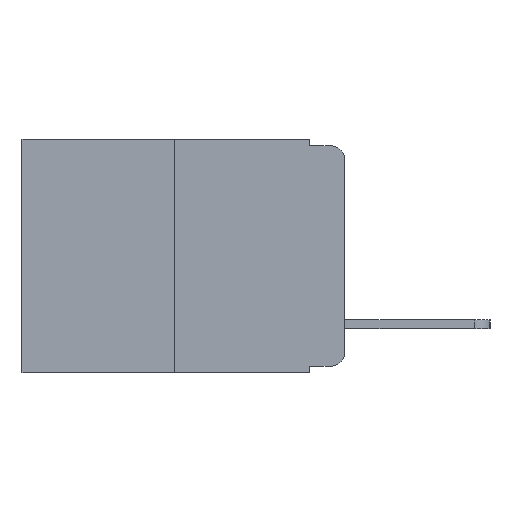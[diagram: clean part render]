
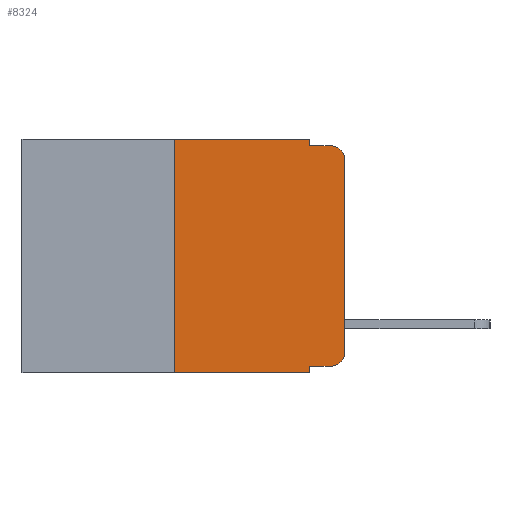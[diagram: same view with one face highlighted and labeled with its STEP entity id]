
A CAD part, left-side view. The second image highlights one B-rep face of the part: STEP entity #8324.
In plain terms, the highlighted planar face has unit normal (-1, 0, 0).
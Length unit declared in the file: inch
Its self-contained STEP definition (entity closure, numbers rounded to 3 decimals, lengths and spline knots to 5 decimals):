
#100 = CARTESIAN_POINT ( 'NONE',  ( 0., 0.051, -0.333 ) ) ;
#491 = VERTEX_POINT ( 'NONE', #8884 ) ;
#670 = VERTEX_POINT ( 'NONE', #9890 ) ;
#972 = VECTOR ( 'NONE', #1448, 39.37008 ) ;
#1049 = EDGE_CURVE ( 'NONE', #491, #8354, #5677, .T. ) ;
#1166 = LINE ( 'NONE', #12088, #6371 ) ;
#1448 = DIRECTION ( 'NONE',  ( 0., 0., 1. ) ) ;
#1479 = VECTOR ( 'NONE', #1860, 39.37008 ) ;
#1709 = PLANE ( 'NONE',  #5831 ) ;
#1791 = VERTEX_POINT ( 'NONE', #10513 ) ;
#1794 = VECTOR ( 'NONE', #8146, 39.37008 ) ;
#1860 = DIRECTION ( 'NONE',  ( 0., -1., 0. ) ) ;
#1942 = AXIS2_PLACEMENT_3D ( 'NONE', #11087, #5425, #11961 ) ;
#1957 = VECTOR ( 'NONE', #8129, 39.37008 ) ;
#1974 = EDGE_CURVE ( 'NONE', #1791, #10375, #2445, .T. ) ;
#2292 = LINE ( 'NONE', #7148, #12209 ) ;
#2402 = LINE ( 'NONE', #7949, #9971 ) ;
#2424 = ORIENTED_EDGE ( 'NONE', *, *, #10102, .T. ) ;
#2445 = CIRCLE ( 'NONE', #5504, 0.02 ) ;
#2684 = EDGE_CURVE ( 'NONE', #4507, #1791, #2402, .T. ) ;
#2780 = DIRECTION ( 'NONE',  ( 0., 0., -1. ) ) ;
#2944 = ORIENTED_EDGE ( 'NONE', *, *, #4035, .F. ) ;
#2957 = VECTOR ( 'NONE', #10579, 39.37008 ) ;
#3113 = DIRECTION ( 'NONE',  ( 0., 0., -1. ) ) ;
#3202 = ORIENTED_EDGE ( 'NONE', *, *, #3351, .F. ) ;
#3351 = EDGE_CURVE ( 'NONE', #4507, #4591, #1166, .T. ) ;
#3646 = ORIENTED_EDGE ( 'NONE', *, *, #1049, .F. ) ;
#3721 = ORIENTED_EDGE ( 'NONE', *, *, #11720, .T. ) ;
#3833 = CARTESIAN_POINT ( 'NONE',  ( 0., 0.051, 0. ) ) ;
#4035 = EDGE_CURVE ( 'NONE', #6986, #491, #11165, .T. ) ;
#4389 = CARTESIAN_POINT ( 'NONE',  ( 0., 0.02, -0.313 ) ) ;
#4422 = CARTESIAN_POINT ( 'NONE',  ( 0., 0., -0.313 ) ) ;
#4507 = VERTEX_POINT ( 'NONE', #100 ) ;
#4591 = VERTEX_POINT ( 'NONE', #7546 ) ;
#5425 = DIRECTION ( 'NONE',  ( -1., 0., 0. ) ) ;
#5504 = AXIS2_PLACEMENT_3D ( 'NONE', #4389, #8541, #8479 ) ;
#5677 = LINE ( 'NONE', #8475, #2957 ) ;
#5831 = AXIS2_PLACEMENT_3D ( 'NONE', #11436, #8782, #2780 ) ;
#6112 = EDGE_CURVE ( 'NONE', #8354, #11029, #2292, .T. ) ;
#6114 = ORIENTED_EDGE ( 'NONE', *, *, #2684, .T. ) ;
#6132 = ORIENTED_EDGE ( 'NONE', *, *, #8092, .T. ) ;
#6163 = CARTESIAN_POINT ( 'NONE',  ( 0., 0.051, -0.01 ) ) ;
#6369 = ORIENTED_EDGE ( 'NONE', *, *, #1974, .T. ) ;
#6371 = VECTOR ( 'NONE', #10505, 39.37008 ) ;
#6565 = DIRECTION ( 'NONE',  ( 0., -1., 0. ) ) ;
#6590 = CARTESIAN_POINT ( 'NONE',  ( 0., 0.25, 0. ) ) ;
#6633 = LINE ( 'NONE', #12437, #1479 ) ;
#6772 = EDGE_CURVE ( 'NONE', #11029, #670, #9754, .T. ) ;
#6856 = EDGE_LOOP ( 'NONE', ( #3721, #6132, #10004, #7521, #3646, #2944, #2424, #3202, #6114, #6369 ) ) ;
#6986 = VERTEX_POINT ( 'NONE', #11988 ) ;
#7148 = CARTESIAN_POINT ( 'NONE',  ( 0., 0.051, 0. ) ) ;
#7205 = CIRCLE ( 'NONE', #1942, 0.02 ) ;
#7376 = LINE ( 'NONE', #9073, #1957 ) ;
#7521 = ORIENTED_EDGE ( 'NONE', *, *, #6112, .F. ) ;
#7546 = CARTESIAN_POINT ( 'NONE',  ( 0., 0.051, -0.343 ) ) ;
#7949 = CARTESIAN_POINT ( 'NONE',  ( 0., 0.051, -0.333 ) ) ;
#8092 = EDGE_CURVE ( 'NONE', #12553, #670, #7205, .T. ) ;
#8129 = DIRECTION ( 'NONE',  ( 0., 0., 1. ) ) ;
#8146 = DIRECTION ( 'NONE',  ( 0., -1., 0. ) ) ;
#8324 = ADVANCED_FACE ( 'NONE', ( #11644 ), #1709, .F. ) ;
#8354 = VERTEX_POINT ( 'NONE', #3833 ) ;
#8475 = CARTESIAN_POINT ( 'NONE',  ( 0., 0.473, 0. ) ) ;
#8479 = DIRECTION ( 'NONE',  ( 0., 0., -1. ) ) ;
#8541 = DIRECTION ( 'NONE',  ( -1., 0., 0. ) ) ;
#8782 = DIRECTION ( 'NONE',  ( 1., 0., 0. ) ) ;
#8884 = CARTESIAN_POINT ( 'NONE',  ( 0., 0.25, 0. ) ) ;
#9073 = CARTESIAN_POINT ( 'NONE',  ( 0., 0., 0. ) ) ;
#9754 = LINE ( 'NONE', #6163, #1794 ) ;
#9890 = CARTESIAN_POINT ( 'NONE',  ( 0., 0.02, -0.01 ) ) ;
#9971 = VECTOR ( 'NONE', #6565, 39.37008 ) ;
#10004 = ORIENTED_EDGE ( 'NONE', *, *, #6772, .F. ) ;
#10102 = EDGE_CURVE ( 'NONE', #6986, #4591, #6633, .T. ) ;
#10112 = CARTESIAN_POINT ( 'NONE',  ( 0., 0.051, -0.01 ) ) ;
#10375 = VERTEX_POINT ( 'NONE', #4422 ) ;
#10505 = DIRECTION ( 'NONE',  ( 0., 0., -1. ) ) ;
#10513 = CARTESIAN_POINT ( 'NONE',  ( 0., 0.02, -0.333 ) ) ;
#10520 = CARTESIAN_POINT ( 'NONE',  ( 0., 0., -0.03 ) ) ;
#10579 = DIRECTION ( 'NONE',  ( 0., -1., 0. ) ) ;
#11029 = VERTEX_POINT ( 'NONE', #10112 ) ;
#11087 = CARTESIAN_POINT ( 'NONE',  ( 0., 0.02, -0.03 ) ) ;
#11165 = LINE ( 'NONE', #6590, #972 ) ;
#11436 = CARTESIAN_POINT ( 'NONE',  ( 0., 0.473, 0. ) ) ;
#11644 = FACE_OUTER_BOUND ( 'NONE', #6856, .T. ) ;
#11720 = EDGE_CURVE ( 'NONE', #10375, #12553, #7376, .T. ) ;
#11961 = DIRECTION ( 'NONE',  ( 0., 0., -1. ) ) ;
#11988 = CARTESIAN_POINT ( 'NONE',  ( 0., 0.25, -0.343 ) ) ;
#12088 = CARTESIAN_POINT ( 'NONE',  ( 0., 0.051, 0. ) ) ;
#12209 = VECTOR ( 'NONE', #3113, 39.37008 ) ;
#12437 = CARTESIAN_POINT ( 'NONE',  ( 0., 0.473, -0.343 ) ) ;
#12553 = VERTEX_POINT ( 'NONE', #10520 ) ;
